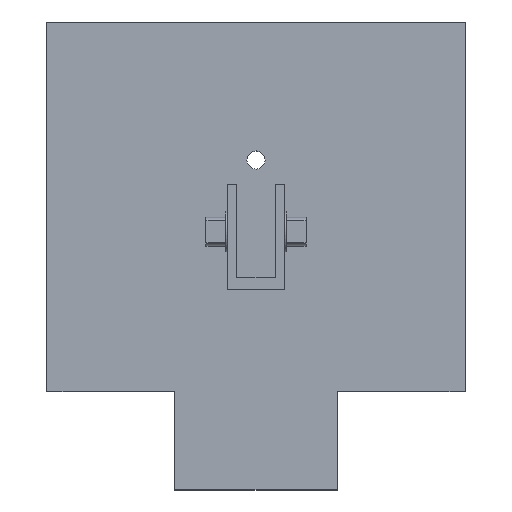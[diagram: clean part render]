
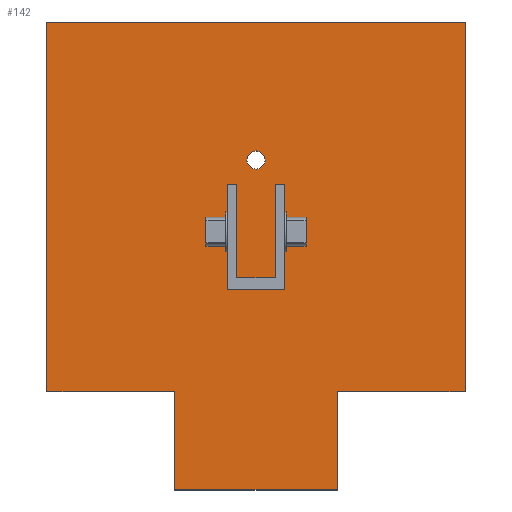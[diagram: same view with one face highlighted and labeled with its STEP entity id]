
A CAD part, top view. The second image highlights one B-rep face of the part: STEP entity #142.
In plain terms, the highlighted planar face has unit normal (0, 0, 1).
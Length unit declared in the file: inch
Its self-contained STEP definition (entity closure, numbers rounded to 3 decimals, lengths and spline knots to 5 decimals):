
#3 = VERTEX_POINT ( 'NONE', #561 ) ;
#35 = CARTESIAN_POINT ( 'NONE',  ( 1.74, 0., 1.5 ) ) ;
#46 = CARTESIAN_POINT ( 'NONE',  ( 0., 3.2646, 1.5 ) ) ;
#54 = VECTOR ( 'NONE', #829, 39.37008 ) ;
#63 = VERTEX_POINT ( 'NONE', #299 ) ;
#72 = EDGE_CURVE ( 'NONE', #166, #889, #1161, .T. ) ;
#78 = LINE ( 'NONE', #276, #898 ) ;
#80 = EDGE_CURVE ( 'NONE', #701, #3, #1127, .T. ) ;
#88 = EDGE_CURVE ( 'NONE', #1165, #1039, #1160, .T. ) ;
#95 = ORIENTED_EDGE ( 'NONE', *, *, #530, .F. ) ;
#128 = CARTESIAN_POINT ( 'NONE',  ( 0., 3.2646, 1.5 ) ) ;
#133 = CARTESIAN_POINT ( 'NONE',  ( 0., 0., 1.5 ) ) ;
#142 = ADVANCED_FACE ( 'NONE', ( #841, #1054, #553 ), #616, .T. ) ;
#149 = DIRECTION ( 'NONE',  ( 1., 0., 0. ) ) ;
#150 = LINE ( 'NONE', #128, #54 ) ;
#154 = EDGE_LOOP ( 'NONE', ( #369, #1182, #770, #198, #463, #162, #1043, #1005 ) ) ;
#159 = EDGE_CURVE ( 'NONE', #3, #724, #741, .T. ) ;
#162 = ORIENTED_EDGE ( 'NONE', *, *, #663, .T. ) ;
#166 = VERTEX_POINT ( 'NONE', #931 ) ;
#174 = EDGE_CURVE ( 'NONE', #904, #1111, #295, .T. ) ;
#198 = ORIENTED_EDGE ( 'NONE', *, *, #689, .T. ) ;
#209 = CARTESIAN_POINT ( 'NONE',  ( 1.74, 1.05, 1.5 ) ) ;
#254 = EDGE_CURVE ( 'NONE', #459, #63, #78, .T. ) ;
#264 = LINE ( 'NONE', #1007, #951 ) ;
#267 = VECTOR ( 'NONE', #942, 39.37008 ) ;
#276 = CARTESIAN_POINT ( 'NONE',  ( 0., 0., 1.5 ) ) ;
#283 = VERTEX_POINT ( 'NONE', #560 ) ;
#291 = AXIS2_PLACEMENT_3D ( 'NONE', #133, #938, #720 ) ;
#295 = LINE ( 'NONE', #35, #914 ) ;
#299 = CARTESIAN_POINT ( 'NONE',  ( 0., 1.05, 1.5 ) ) ;
#316 = CARTESIAN_POINT ( 'NONE',  ( 0.56508, 0., 1.5 ) ) ;
#320 = VERTEX_POINT ( 'NONE', #976 ) ;
#329 = CARTESIAN_POINT ( 'NONE',  ( 1.74, 0., 1.5 ) ) ;
#338 = CARTESIAN_POINT ( 'NONE',  ( 3.105, 0., 1.5 ) ) ;
#367 = ORIENTED_EDGE ( 'NONE', *, *, #1049, .T. ) ;
#369 = ORIENTED_EDGE ( 'NONE', *, *, #562, .T. ) ;
#375 = EDGE_CURVE ( 'NONE', #889, #166, #958, .T. ) ;
#384 = DIRECTION ( 'NONE',  ( 0., 0., 1. ) ) ;
#387 = AXIS2_PLACEMENT_3D ( 'NONE', #1192, #384, #1006 ) ;
#401 = CARTESIAN_POINT ( 'NONE',  ( 1.17492, 3.2646, 1.5 ) ) ;
#405 = CARTESIAN_POINT ( 'NONE',  ( 0., 2.2646, 1.5 ) ) ;
#419 = DIRECTION ( 'NONE',  ( -1., 0., 0. ) ) ;
#420 = DIRECTION ( 'NONE',  ( 1., 0., 0. ) ) ;
#431 = EDGE_CURVE ( 'NONE', #320, #701, #817, .T. ) ;
#447 = CARTESIAN_POINT ( 'NONE',  ( 3.105, 1.05, 1.5 ) ) ;
#455 = LINE ( 'NONE', #869, #1278 ) ;
#457 = VECTOR ( 'NONE', #785, 39.37008 ) ;
#459 = VERTEX_POINT ( 'NONE', #578 ) ;
#463 = ORIENTED_EDGE ( 'NONE', *, *, #1187, .T. ) ;
#481 = DIRECTION ( 'NONE',  ( 0., 1., 0. ) ) ;
#488 = CARTESIAN_POINT ( 'NONE',  ( -1.365, 0., 1.5 ) ) ;
#495 = EDGE_CURVE ( 'NONE', #633, #977, #996, .T. ) ;
#499 = AXIS2_PLACEMENT_3D ( 'NONE', #804, #509, #420 ) ;
#503 = ORIENTED_EDGE ( 'NONE', *, *, #431, .F. ) ;
#507 = CARTESIAN_POINT ( 'NONE',  ( 0.56508, 2.13941, 1.5 ) ) ;
#509 = DIRECTION ( 'NONE',  ( 0., 0., 1. ) ) ;
#515 = VECTOR ( 'NONE', #419, 39.37008 ) ;
#530 = EDGE_CURVE ( 'NONE', #724, #1111, #1254, .T. ) ;
#533 = EDGE_CURVE ( 'NONE', #633, #962, #1036, .T. ) ;
#547 = ORIENTED_EDGE ( 'NONE', *, *, #1285, .F. ) ;
#553 = FACE_OUTER_BOUND ( 'NONE', #742, .T. ) ;
#560 = CARTESIAN_POINT ( 'NONE',  ( 1.17492, 2.13941, 1.5 ) ) ;
#561 = CARTESIAN_POINT ( 'NONE',  ( 3.105, 5., 1.5 ) ) ;
#562 = EDGE_CURVE ( 'NONE', #798, #962, #1052, .T. ) ;
#564 = LINE ( 'NONE', #733, #267 ) ;
#571 = CARTESIAN_POINT ( 'NONE',  ( 0.56508, 3.2646, 1.5 ) ) ;
#578 = CARTESIAN_POINT ( 'NONE',  ( 0., 0., 1.5 ) ) ;
#581 = DIRECTION ( 'NONE',  ( 1., 0., 0. ) ) ;
#592 = ORIENTED_EDGE ( 'NONE', *, *, #80, .F. ) ;
#593 = CARTESIAN_POINT ( 'NONE',  ( 1.07492, 2.2646, 1.5 ) ) ;
#599 = DIRECTION ( 'NONE',  ( 0., 1., 0. ) ) ;
#616 = PLANE ( 'NONE',  #291 ) ;
#622 = DIRECTION ( 'NONE',  ( 0., 1., 0. ) ) ;
#633 = VERTEX_POINT ( 'NONE', #593 ) ;
#663 = EDGE_CURVE ( 'NONE', #283, #1165, #564, .T. ) ;
#689 = EDGE_CURVE ( 'NONE', #977, #1062, #150, .T. ) ;
#700 = CARTESIAN_POINT ( 'NONE',  ( 0., 1.05, 1.5 ) ) ;
#701 = VERTEX_POINT ( 'NONE', #935 ) ;
#720 = DIRECTION ( 'NONE',  ( 1., 0., 0. ) ) ;
#724 = VERTEX_POINT ( 'NONE', #447 ) ;
#733 = CARTESIAN_POINT ( 'NONE',  ( 0., 2.13941, 1.5 ) ) ;
#741 = LINE ( 'NONE', #338, #819 ) ;
#742 = EDGE_LOOP ( 'NONE', ( #1109, #592, #503, #547, #899, #367, #940, #95 ) ) ;
#746 = CARTESIAN_POINT ( 'NONE',  ( 0.66508, 2.2646, 1.5 ) ) ;
#760 = DIRECTION ( 'NONE',  ( 0., 1., 0. ) ) ;
#770 = ORIENTED_EDGE ( 'NONE', *, *, #495, .T. ) ;
#785 = DIRECTION ( 'NONE',  ( 0., 1., 0. ) ) ;
#798 = VERTEX_POINT ( 'NONE', #1035 ) ;
#801 = DIRECTION ( 'NONE',  ( 1., 0., 0. ) ) ;
#804 = CARTESIAN_POINT ( 'NONE',  ( 0.87, 3.5246, 1.5 ) ) ;
#809 = CARTESIAN_POINT ( 'NONE',  ( 0.66508, 0., 1.5 ) ) ;
#817 = LINE ( 'NONE', #488, #1104 ) ;
#819 = VECTOR ( 'NONE', #1131, 39.37008 ) ;
#829 = DIRECTION ( 'NONE',  ( 1., 0., 0. ) ) ;
#841 = FACE_BOUND ( 'NONE', #154, .T. ) ;
#856 = EDGE_CURVE ( 'NONE', #1039, #798, #1138, .T. ) ;
#869 = CARTESIAN_POINT ( 'NONE',  ( 0., 1.05, 1.5 ) ) ;
#889 = VERTEX_POINT ( 'NONE', #1263 ) ;
#896 = VECTOR ( 'NONE', #1027, 39.37008 ) ;
#898 = VECTOR ( 'NONE', #760, 39.37008 ) ;
#899 = ORIENTED_EDGE ( 'NONE', *, *, #254, .F. ) ;
#904 = VERTEX_POINT ( 'NONE', #329 ) ;
#907 = DIRECTION ( 'NONE',  ( -1., 0., 0. ) ) ;
#914 = VECTOR ( 'NONE', #622, 39.37008 ) ;
#926 = DIRECTION ( 'NONE',  ( 0., -1., 0. ) ) ;
#929 = CARTESIAN_POINT ( 'NONE',  ( 1.17492, 0., 1.5 ) ) ;
#931 = CARTESIAN_POINT ( 'NONE',  ( 0.9671, 3.5246, 1.5 ) ) ;
#935 = CARTESIAN_POINT ( 'NONE',  ( -1.365, 5., 1.5 ) ) ;
#938 = DIRECTION ( 'NONE',  ( 0., 0., 1. ) ) ;
#940 = ORIENTED_EDGE ( 'NONE', *, *, #174, .T. ) ;
#942 = DIRECTION ( 'NONE',  ( -1., 0., 0. ) ) ;
#951 = VECTOR ( 'NONE', #801, 39.37008 ) ;
#958 = CIRCLE ( 'NONE', #387, 0.0971 ) ;
#962 = VERTEX_POINT ( 'NONE', #746 ) ;
#972 = VECTOR ( 'NONE', #581, 39.37008 ) ;
#976 = CARTESIAN_POINT ( 'NONE',  ( -1.365, 1.05, 1.5 ) ) ;
#977 = VERTEX_POINT ( 'NONE', #1257 ) ;
#984 = ORIENTED_EDGE ( 'NONE', *, *, #375, .F. ) ;
#996 = LINE ( 'NONE', #1301, #457 ) ;
#1000 = ORIENTED_EDGE ( 'NONE', *, *, #72, .F. ) ;
#1005 = ORIENTED_EDGE ( 'NONE', *, *, #856, .T. ) ;
#1006 = DIRECTION ( 'NONE',  ( 1., 0., 0. ) ) ;
#1007 = CARTESIAN_POINT ( 'NONE',  ( 0., 0., 1.5 ) ) ;
#1027 = DIRECTION ( 'NONE',  ( 0., -1., 0. ) ) ;
#1031 = DIRECTION ( 'NONE',  ( -1., 0., 0. ) ) ;
#1035 = CARTESIAN_POINT ( 'NONE',  ( 0.66508, 3.2646, 1.5 ) ) ;
#1036 = LINE ( 'NONE', #405, #515 ) ;
#1039 = VERTEX_POINT ( 'NONE', #571 ) ;
#1043 = ORIENTED_EDGE ( 'NONE', *, *, #88, .T. ) ;
#1049 = EDGE_CURVE ( 'NONE', #459, #904, #264, .T. ) ;
#1052 = LINE ( 'NONE', #809, #1212 ) ;
#1054 = FACE_BOUND ( 'NONE', #1074, .T. ) ;
#1062 = VERTEX_POINT ( 'NONE', #401 ) ;
#1074 = EDGE_LOOP ( 'NONE', ( #1000, #984 ) ) ;
#1077 = VECTOR ( 'NONE', #149, 39.37008 ) ;
#1104 = VECTOR ( 'NONE', #481, 39.37008 ) ;
#1109 = ORIENTED_EDGE ( 'NONE', *, *, #159, .F. ) ;
#1111 = VERTEX_POINT ( 'NONE', #209 ) ;
#1127 = LINE ( 'NONE', #1205, #972 ) ;
#1131 = DIRECTION ( 'NONE',  ( 0., -1., 0. ) ) ;
#1138 = LINE ( 'NONE', #46, #1077 ) ;
#1143 = VECTOR ( 'NONE', #599, 39.37008 ) ;
#1160 = LINE ( 'NONE', #316, #1143 ) ;
#1161 = CIRCLE ( 'NONE', #499, 0.0971 ) ;
#1165 = VERTEX_POINT ( 'NONE', #507 ) ;
#1182 = ORIENTED_EDGE ( 'NONE', *, *, #533, .F. ) ;
#1187 = EDGE_CURVE ( 'NONE', #1062, #283, #1309, .T. ) ;
#1192 = CARTESIAN_POINT ( 'NONE',  ( 0.87, 3.5246, 1.5 ) ) ;
#1205 = CARTESIAN_POINT ( 'NONE',  ( 0., 5., 1.5 ) ) ;
#1212 = VECTOR ( 'NONE', #926, 39.37008 ) ;
#1254 = LINE ( 'NONE', #700, #1312 ) ;
#1257 = CARTESIAN_POINT ( 'NONE',  ( 1.07492, 3.2646, 1.5 ) ) ;
#1263 = CARTESIAN_POINT ( 'NONE',  ( 0.7729, 3.5246, 1.5 ) ) ;
#1278 = VECTOR ( 'NONE', #1031, 39.37008 ) ;
#1285 = EDGE_CURVE ( 'NONE', #63, #320, #455, .T. ) ;
#1301 = CARTESIAN_POINT ( 'NONE',  ( 1.07492, 0., 1.5 ) ) ;
#1309 = LINE ( 'NONE', #929, #896 ) ;
#1312 = VECTOR ( 'NONE', #907, 39.37008 ) ;
